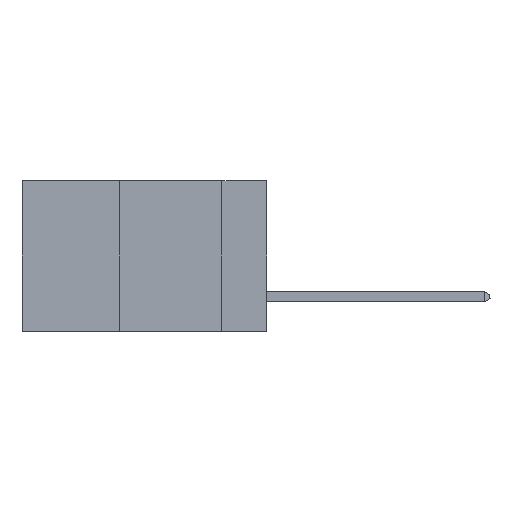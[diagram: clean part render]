
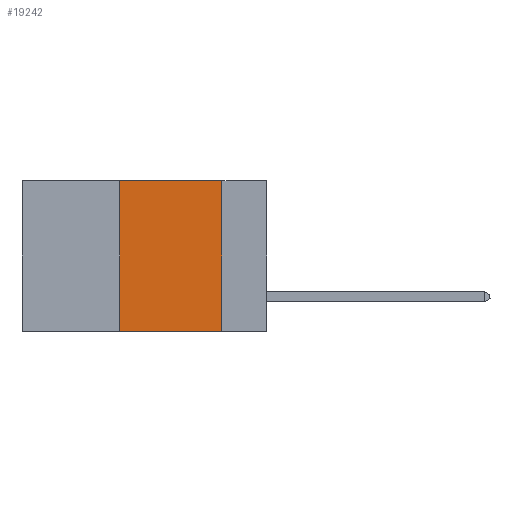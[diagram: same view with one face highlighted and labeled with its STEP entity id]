
A CAD part, left-side view. The second image highlights one B-rep face of the part: STEP entity #19242.
In plain terms, the highlighted planar face has unit normal (-1, 0, 0).
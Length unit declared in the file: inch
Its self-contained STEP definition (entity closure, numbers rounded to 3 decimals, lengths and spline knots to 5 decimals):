
#791 = CARTESIAN_POINT ( 'NONE',  ( 0., 0.6, 0. ) ) ;
#4027 = VECTOR ( 'NONE', #43458, 39.37008 ) ;
#5375 = ORIENTED_EDGE ( 'NONE', *, *, #9448, .T. ) ;
#8410 = CARTESIAN_POINT ( 'NONE',  ( 0., 0.36, 0. ) ) ;
#9321 = DIRECTION ( 'NONE',  ( 1., 0., 0. ) ) ;
#9448 = EDGE_CURVE ( 'NONE', #29322, #35134, #41601, .T. ) ;
#10813 = CARTESIAN_POINT ( 'NONE',  ( 0., 0.11, 0. ) ) ;
#11388 = ORIENTED_EDGE ( 'NONE', *, *, #29137, .F. ) ;
#11630 = LINE ( 'NONE', #791, #4027 ) ;
#11774 = VECTOR ( 'NONE', #31883, 39.37008 ) ;
#15914 = DIRECTION ( 'NONE',  ( 0., 0., 1. ) ) ;
#19242 = ADVANCED_FACE ( 'NONE', ( #48033 ), #32316, .F. ) ;
#20420 = CARTESIAN_POINT ( 'NONE',  ( 0., 0.6, 0. ) ) ;
#22503 = VERTEX_POINT ( 'NONE', #10813 ) ;
#23158 = CARTESIAN_POINT ( 'NONE',  ( 0., 0.36, 0. ) ) ;
#28296 = ORIENTED_EDGE ( 'NONE', *, *, #41501, .F. ) ;
#29137 = EDGE_CURVE ( 'NONE', #22503, #35134, #42954, .T. ) ;
#29322 = VERTEX_POINT ( 'NONE', #44222 ) ;
#30561 = CARTESIAN_POINT ( 'NONE',  ( 0., 0.11, -0.37 ) ) ;
#31567 = EDGE_CURVE ( 'NONE', #29322, #48420, #42172, .T. ) ;
#31883 = DIRECTION ( 'NONE',  ( 0., -1., 0. ) ) ;
#32316 = PLANE ( 'NONE',  #36727 ) ;
#32357 = VECTOR ( 'NONE', #15914, 39.37008 ) ;
#33386 = EDGE_LOOP ( 'NONE', ( #11388, #28296, #45367, #5375 ) ) ;
#33575 = DIRECTION ( 'NONE',  ( 0., 0., -1. ) ) ;
#35134 = VERTEX_POINT ( 'NONE', #30561 ) ;
#36727 = AXIS2_PLACEMENT_3D ( 'NONE', #20420, #9321, #46567 ) ;
#41501 = EDGE_CURVE ( 'NONE', #48420, #22503, #11630, .T. ) ;
#41601 = LINE ( 'NONE', #47042, #11774 ) ;
#42172 = LINE ( 'NONE', #8410, #32357 ) ;
#42954 = LINE ( 'NONE', #48382, #44179 ) ;
#43458 = DIRECTION ( 'NONE',  ( 0., -1., 0. ) ) ;
#44179 = VECTOR ( 'NONE', #33575, 39.37008 ) ;
#44222 = CARTESIAN_POINT ( 'NONE',  ( 0., 0.36, -0.37 ) ) ;
#45367 = ORIENTED_EDGE ( 'NONE', *, *, #31567, .F. ) ;
#46567 = DIRECTION ( 'NONE',  ( 0., 0., -1. ) ) ;
#47042 = CARTESIAN_POINT ( 'NONE',  ( 0., 0.6, -0.37 ) ) ;
#48033 = FACE_OUTER_BOUND ( 'NONE', #33386, .T. ) ;
#48382 = CARTESIAN_POINT ( 'NONE',  ( 0., 0.11, 0. ) ) ;
#48420 = VERTEX_POINT ( 'NONE', #23158 ) ;
